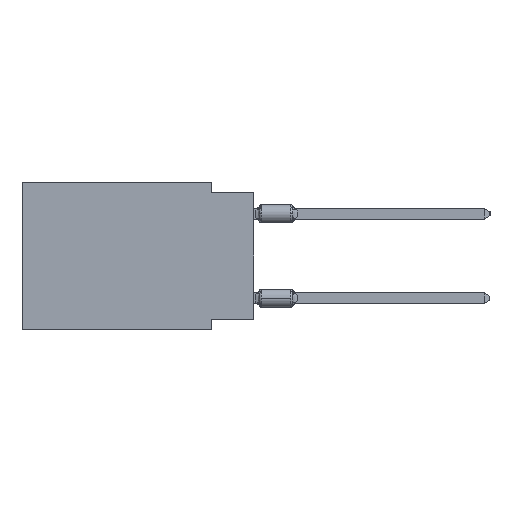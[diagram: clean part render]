
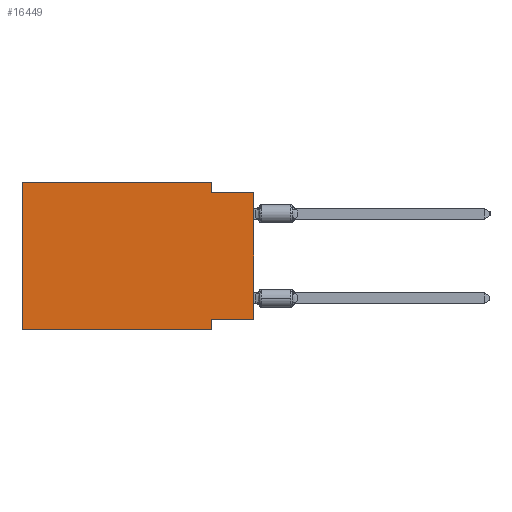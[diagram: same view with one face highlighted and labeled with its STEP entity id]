
A CAD part, left-side view. The second image highlights one B-rep face of the part: STEP entity #16449.
In plain terms, the highlighted planar face has unit normal (-1, 0, 0).
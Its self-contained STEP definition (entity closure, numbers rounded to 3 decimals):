
#62 = ORIENTED_EDGE ( 'NONE', *, *, #8594, .F. ) ;
#624 = CARTESIAN_POINT ( 'NONE',  ( 0., 2.54, -0.635 ) ) ;
#1297 = VECTOR ( 'NONE', #27219, 1000. ) ;
#1433 = LINE ( 'NONE', #8909, #1297 ) ;
#1510 = DIRECTION ( 'NONE',  ( 0., -1., 0. ) ) ;
#1727 = VERTEX_POINT ( 'NONE', #33407 ) ;
#4669 = DIRECTION ( 'NONE',  ( 0., -1., 0. ) ) ;
#5797 = EDGE_CURVE ( 'NONE', #10632, #1727, #6437, .T. ) ;
#6437 = LINE ( 'NONE', #27463, #20636 ) ;
#7218 = CARTESIAN_POINT ( 'NONE',  ( 0., 2.54, -8.255 ) ) ;
#7460 = DIRECTION ( 'NONE',  ( 0., 0., 1. ) ) ;
#7785 = EDGE_CURVE ( 'NONE', #31433, #12393, #1433, .T. ) ;
#8022 = LINE ( 'NONE', #8183, #33440 ) ;
#8028 = CARTESIAN_POINT ( 'NONE',  ( 0., 0., -0.635 ) ) ;
#8183 = CARTESIAN_POINT ( 'NONE',  ( 0., 2.54, -8.89 ) ) ;
#8390 = DIRECTION ( 'NONE',  ( 0., 0., -1. ) ) ;
#8594 = EDGE_CURVE ( 'NONE', #31433, #10632, #32921, .T. ) ;
#8909 = CARTESIAN_POINT ( 'NONE',  ( 0., 13.97, -8.89 ) ) ;
#10217 = VECTOR ( 'NONE', #28716, 1000. ) ;
#10326 = CARTESIAN_POINT ( 'NONE',  ( 0., 13.97, 0. ) ) ;
#10632 = VERTEX_POINT ( 'NONE', #17728 ) ;
#11725 = VECTOR ( 'NONE', #4669, 1000. ) ;
#11846 = AXIS2_PLACEMENT_3D ( 'NONE', #21619, #29419, #8390 ) ;
#12393 = VERTEX_POINT ( 'NONE', #20053 ) ;
#12961 = CARTESIAN_POINT ( 'NONE',  ( 0., 2.54, 0. ) ) ;
#15484 = ORIENTED_EDGE ( 'NONE', *, *, #27318, .F. ) ;
#15742 = ORIENTED_EDGE ( 'NONE', *, *, #27829, .F. ) ;
#16449 = ADVANCED_FACE ( 'NONE', ( #32141 ), #29769, .F. ) ;
#16722 = EDGE_CURVE ( 'NONE', #26431, #19740, #26153, .T. ) ;
#17384 = CARTESIAN_POINT ( 'NONE',  ( 0., 0., -0.635 ) ) ;
#17728 = CARTESIAN_POINT ( 'NONE',  ( 0., 13.97, 0. ) ) ;
#17879 = LINE ( 'NONE', #12961, #19343 ) ;
#18830 = DIRECTION ( 'NONE',  ( 0., 1., 0. ) ) ;
#18916 = ORIENTED_EDGE ( 'NONE', *, *, #16722, .T. ) ;
#19343 = VECTOR ( 'NONE', #28227, 1000. ) ;
#19647 = VECTOR ( 'NONE', #7460, 1000. ) ;
#19740 = VERTEX_POINT ( 'NONE', #8028 ) ;
#19795 = VECTOR ( 'NONE', #18830, 1000. ) ;
#20053 = CARTESIAN_POINT ( 'NONE',  ( 0., 2.54, -8.89 ) ) ;
#20340 = CARTESIAN_POINT ( 'NONE',  ( 0., 13.97, -8.89 ) ) ;
#20636 = VECTOR ( 'NONE', #1510, 1000. ) ;
#20925 = ORIENTED_EDGE ( 'NONE', *, *, #28428, .F. ) ;
#21248 = VERTEX_POINT ( 'NONE', #7218 ) ;
#21619 = CARTESIAN_POINT ( 'NONE',  ( 0., 13.97, 0. ) ) ;
#25734 = CARTESIAN_POINT ( 'NONE',  ( 0., 0., -8.255 ) ) ;
#26065 = VERTEX_POINT ( 'NONE', #624 ) ;
#26153 = LINE ( 'NONE', #33324, #10217 ) ;
#26431 = VERTEX_POINT ( 'NONE', #25734 ) ;
#27046 = ORIENTED_EDGE ( 'NONE', *, *, #5797, .F. ) ;
#27219 = DIRECTION ( 'NONE',  ( 0., -1., 0. ) ) ;
#27318 = EDGE_CURVE ( 'NONE', #26431, #21248, #32710, .T. ) ;
#27463 = CARTESIAN_POINT ( 'NONE',  ( 0., 13.97, 0. ) ) ;
#27487 = EDGE_LOOP ( 'NONE', ( #18916, #15742, #28491, #27046, #62, #30448, #20925, #15484 ) ) ;
#27736 = LINE ( 'NONE', #17384, #11725 ) ;
#27829 = EDGE_CURVE ( 'NONE', #26065, #19740, #27736, .T. ) ;
#28227 = DIRECTION ( 'NONE',  ( 0., 0., -1. ) ) ;
#28308 = EDGE_CURVE ( 'NONE', #1727, #26065, #17879, .T. ) ;
#28428 = EDGE_CURVE ( 'NONE', #21248, #12393, #8022, .T. ) ;
#28491 = ORIENTED_EDGE ( 'NONE', *, *, #28308, .F. ) ;
#28716 = DIRECTION ( 'NONE',  ( 0., 0., 1. ) ) ;
#29199 = CARTESIAN_POINT ( 'NONE',  ( 0., 0., -8.255 ) ) ;
#29419 = DIRECTION ( 'NONE',  ( 1., 0., 0. ) ) ;
#29769 = PLANE ( 'NONE',  #11846 ) ;
#30448 = ORIENTED_EDGE ( 'NONE', *, *, #7785, .T. ) ;
#31433 = VERTEX_POINT ( 'NONE', #20340 ) ;
#31598 = DIRECTION ( 'NONE',  ( 0., 0., -1. ) ) ;
#32141 = FACE_OUTER_BOUND ( 'NONE', #27487, .T. ) ;
#32710 = LINE ( 'NONE', #29199, #19795 ) ;
#32921 = LINE ( 'NONE', #10326, #19647 ) ;
#33324 = CARTESIAN_POINT ( 'NONE',  ( 0., 0., 0. ) ) ;
#33407 = CARTESIAN_POINT ( 'NONE',  ( 0., 2.54, 0. ) ) ;
#33440 = VECTOR ( 'NONE', #31598, 1000. ) ;
